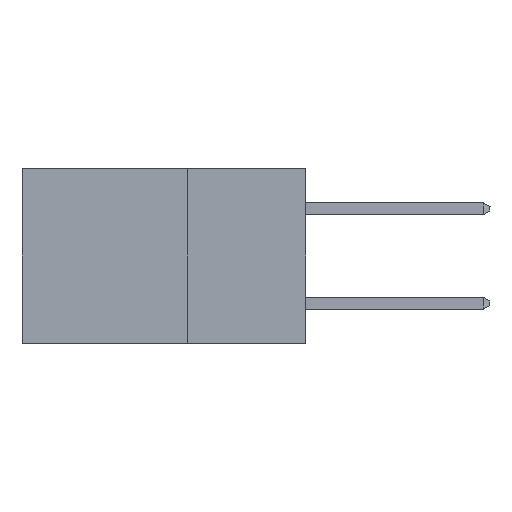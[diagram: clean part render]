
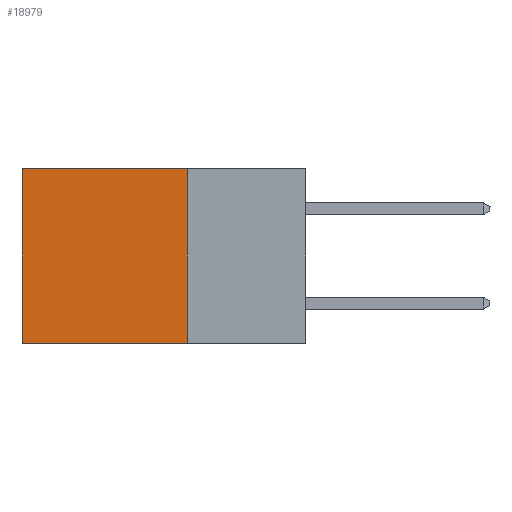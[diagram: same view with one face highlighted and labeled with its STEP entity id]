
A CAD part, left-side view. The second image highlights one B-rep face of the part: STEP entity #18979.
In plain terms, the highlighted planar face has unit normal (-1, 0, 0).
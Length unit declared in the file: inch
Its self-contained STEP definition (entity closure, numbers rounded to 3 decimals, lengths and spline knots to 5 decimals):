
#1540 = DIRECTION ( 'NONE',  ( 0., 0., -1. ) ) ;
#2719 = LINE ( 'NONE', #9998, #8646 ) ;
#2773 = CARTESIAN_POINT ( 'NONE',  ( 0.298, 0.25, 0. ) ) ;
#3321 = DIRECTION ( 'NONE',  ( 1., 0., 0. ) ) ;
#4119 = CARTESIAN_POINT ( 'NONE',  ( 0.298, 0.25, 0. ) ) ;
#4642 = EDGE_CURVE ( 'NONE', #8128, #9756, #5528, .T. ) ;
#4663 = VERTEX_POINT ( 'NONE', #17441 ) ;
#5096 = CARTESIAN_POINT ( 'NONE',  ( 0.298, 0.6, -0.37 ) ) ;
#5367 = CARTESIAN_POINT ( 'NONE',  ( 0.298, 0.25, -0.37 ) ) ;
#5528 = LINE ( 'NONE', #12559, #8735 ) ;
#6200 = LINE ( 'NONE', #5367, #16978 ) ;
#6343 = EDGE_CURVE ( 'NONE', #9756, #9974, #6200, .T. ) ;
#6430 = FACE_OUTER_BOUND ( 'NONE', #13638, .T. ) ;
#6621 = EDGE_CURVE ( 'NONE', #4663, #9974, #2719, .T. ) ;
#7260 = CARTESIAN_POINT ( 'NONE',  ( 0.298, 0.25, -0.37 ) ) ;
#7717 = ORIENTED_EDGE ( 'NONE', *, *, #6621, .T. ) ;
#8128 = VERTEX_POINT ( 'NONE', #4119 ) ;
#8646 = VECTOR ( 'NONE', #14979, 39.37008 ) ;
#8735 = VECTOR ( 'NONE', #1540, 39.37008 ) ;
#8836 = LINE ( 'NONE', #2773, #17165 ) ;
#8955 = ORIENTED_EDGE ( 'NONE', *, *, #4642, .F. ) ;
#9682 = DIRECTION ( 'NONE',  ( 0., 0., -1. ) ) ;
#9756 = VERTEX_POINT ( 'NONE', #7260 ) ;
#9974 = VERTEX_POINT ( 'NONE', #5096 ) ;
#9998 = CARTESIAN_POINT ( 'NONE',  ( 0.298, 0.6, 0. ) ) ;
#12559 = CARTESIAN_POINT ( 'NONE',  ( 0.298, 0.25, 0. ) ) ;
#13638 = EDGE_LOOP ( 'NONE', ( #7717, #19714, #8955, #14001 ) ) ;
#14001 = ORIENTED_EDGE ( 'NONE', *, *, #14342, .T. ) ;
#14342 = EDGE_CURVE ( 'NONE', #8128, #4663, #8836, .T. ) ;
#14979 = DIRECTION ( 'NONE',  ( 0., 0., -1. ) ) ;
#15120 = DIRECTION ( 'NONE',  ( 0., 1., 0. ) ) ;
#15862 = PLANE ( 'NONE',  #16442 ) ;
#16442 = AXIS2_PLACEMENT_3D ( 'NONE', #19045, #3321, #9682 ) ;
#16978 = VECTOR ( 'NONE', #15120, 39.37008 ) ;
#17165 = VECTOR ( 'NONE', #18487, 39.37008 ) ;
#17441 = CARTESIAN_POINT ( 'NONE',  ( 0.298, 0.6, 0. ) ) ;
#18487 = DIRECTION ( 'NONE',  ( 0., 1., 0. ) ) ;
#18979 = ADVANCED_FACE ( 'NONE', ( #6430 ), #15862, .F. ) ;
#19045 = CARTESIAN_POINT ( 'NONE',  ( 0.298, 0.25, 0. ) ) ;
#19714 = ORIENTED_EDGE ( 'NONE', *, *, #6343, .F. ) ;
